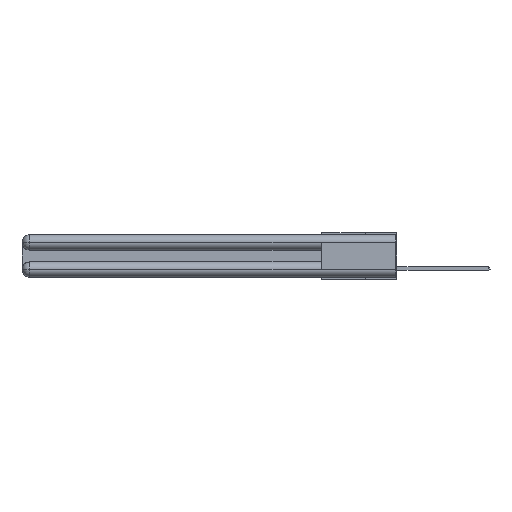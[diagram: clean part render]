
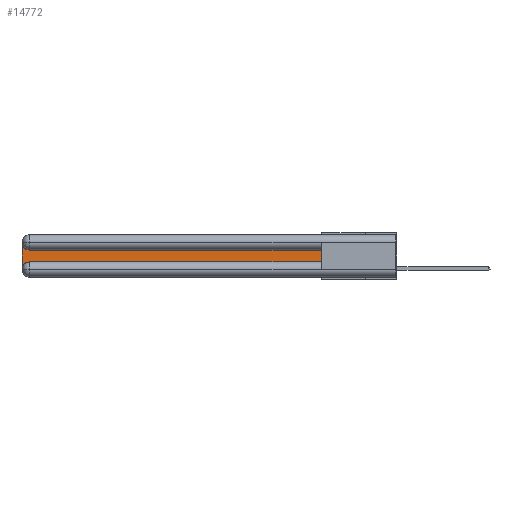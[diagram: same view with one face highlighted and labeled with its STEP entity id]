
A CAD part, left-side view. The second image highlights one B-rep face of the part: STEP entity #14772.
In plain terms, the highlighted planar face has unit normal (-1, 0, 0).
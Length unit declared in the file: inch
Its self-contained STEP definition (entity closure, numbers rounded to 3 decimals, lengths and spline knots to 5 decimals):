
#74 = DIRECTION ( 'NONE',  ( 1., 0., 0. ) ) ;
#305 = CARTESIAN_POINT ( 'NONE',  ( 0.075, 3., -0.2175 ) ) ;
#482 = VECTOR ( 'NONE', #32377, 39.37008 ) ;
#732 = EDGE_CURVE ( 'NONE', #28526, #3916, #10219, .T. ) ;
#823 = EDGE_CURVE ( 'NONE', #26356, #24816, #20213, .T. ) ;
#1279 = LINE ( 'NONE', #11513, #482 ) ;
#1666 = AXIS2_PLACEMENT_3D ( 'NONE', #11751, #32964, #25917 ) ;
#3160 = FACE_OUTER_BOUND ( 'NONE', #33640, .T. ) ;
#3916 = VERTEX_POINT ( 'NONE', #21375 ) ;
#5244 = VERTEX_POINT ( 'NONE', #11298 ) ;
#6644 = CARTESIAN_POINT ( 'NONE',  ( 0.075, 3., -0.2775 ) ) ;
#6675 = ORIENTED_EDGE ( 'NONE', *, *, #8112, .T. ) ;
#7675 = VECTOR ( 'NONE', #19638, 39.37008 ) ;
#8112 = EDGE_CURVE ( 'NONE', #5244, #17555, #21161, .T. ) ;
#8191 = VECTOR ( 'NONE', #14130, 39.37008 ) ;
#8987 = AXIS2_PLACEMENT_3D ( 'NONE', #29275, #18652, #31925 ) ;
#10219 = LINE ( 'NONE', #26122, #19011 ) ;
#10704 = PLANE ( 'NONE',  #8987 ) ;
#11298 = CARTESIAN_POINT ( 'NONE',  ( 0.075, 3., -0.0625 ) ) ;
#11513 = CARTESIAN_POINT ( 'NONE',  ( 0.075, 0.6, -0.2175 ) ) ;
#11751 = CARTESIAN_POINT ( 'NONE',  ( 0.075, 2.94, -0.0625 ) ) ;
#12260 = ORIENTED_EDGE ( 'NONE', *, *, #22263, .T. ) ;
#12766 = ORIENTED_EDGE ( 'NONE', *, *, #25956, .T. ) ;
#14130 = DIRECTION ( 'NONE',  ( 0., 0., -1. ) ) ;
#14301 = EDGE_CURVE ( 'NONE', #17555, #28526, #29017, .T. ) ;
#14483 = CARTESIAN_POINT ( 'NONE',  ( 0.075, 0.6, -0.1225 ) ) ;
#14772 = ADVANCED_FACE ( 'NONE', ( #3160 ), #10704, .F. ) ;
#15151 = CARTESIAN_POINT ( 'NONE',  ( 0.075, 0.6, -0.1225 ) ) ;
#15681 = DIRECTION ( 'NONE',  ( 0., 0., -1. ) ) ;
#15920 = AXIS2_PLACEMENT_3D ( 'NONE', #16149, #74, #15681 ) ;
#16149 = CARTESIAN_POINT ( 'NONE',  ( 0.075, 2.94, -0.2775 ) ) ;
#17555 = VERTEX_POINT ( 'NONE', #6644 ) ;
#18652 = DIRECTION ( 'NONE',  ( 1., 0., 0. ) ) ;
#18930 = CARTESIAN_POINT ( 'NONE',  ( 0.075, 2.94, -0.2175 ) ) ;
#19011 = VECTOR ( 'NONE', #28793, 39.37008 ) ;
#19015 = ORIENTED_EDGE ( 'NONE', *, *, #14301, .T. ) ;
#19638 = DIRECTION ( 'NONE',  ( 0., 1., 0. ) ) ;
#20213 = LINE ( 'NONE', #14483, #7675 ) ;
#21161 = LINE ( 'NONE', #305, #8191 ) ;
#21375 = CARTESIAN_POINT ( 'NONE',  ( 0.075, 0.6, -0.2175 ) ) ;
#22263 = EDGE_CURVE ( 'NONE', #24816, #5244, #27129, .T. ) ;
#24816 = VERTEX_POINT ( 'NONE', #26272 ) ;
#25917 = DIRECTION ( 'NONE',  ( 0., 0., -1. ) ) ;
#25956 = EDGE_CURVE ( 'NONE', #3916, #26356, #1279, .T. ) ;
#26122 = CARTESIAN_POINT ( 'NONE',  ( 0.075, 0.6, -0.2175 ) ) ;
#26272 = CARTESIAN_POINT ( 'NONE',  ( 0.075, 2.94, -0.1225 ) ) ;
#26356 = VERTEX_POINT ( 'NONE', #15151 ) ;
#26683 = ORIENTED_EDGE ( 'NONE', *, *, #823, .T. ) ;
#27129 = CIRCLE ( 'NONE', #1666, 0.06 ) ;
#28526 = VERTEX_POINT ( 'NONE', #18930 ) ;
#28793 = DIRECTION ( 'NONE',  ( 0., -1., 0. ) ) ;
#29017 = CIRCLE ( 'NONE', #15920, 0.06 ) ;
#29275 = CARTESIAN_POINT ( 'NONE',  ( 0.075, 3., -0.1225 ) ) ;
#29571 = ORIENTED_EDGE ( 'NONE', *, *, #732, .T. ) ;
#31925 = DIRECTION ( 'NONE',  ( 0., 0., -1. ) ) ;
#32377 = DIRECTION ( 'NONE',  ( 0., 0., 1. ) ) ;
#32964 = DIRECTION ( 'NONE',  ( 1., 0., 0. ) ) ;
#33640 = EDGE_LOOP ( 'NONE', ( #26683, #12260, #6675, #19015, #29571, #12766 ) ) ;
